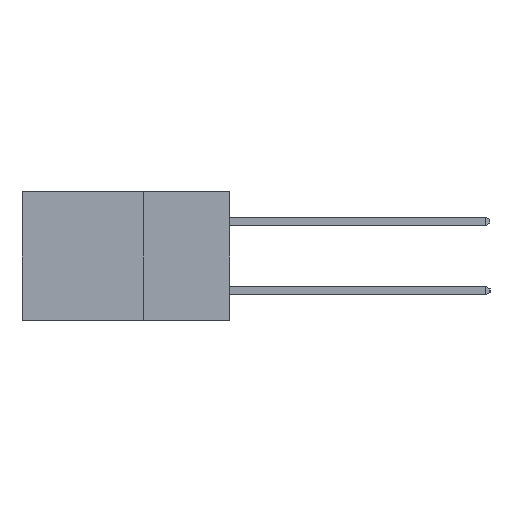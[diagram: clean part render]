
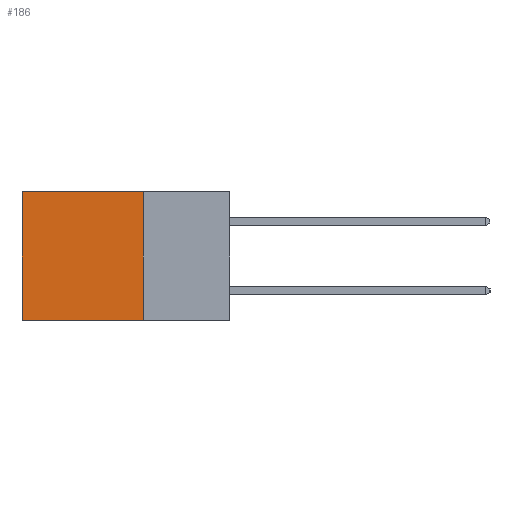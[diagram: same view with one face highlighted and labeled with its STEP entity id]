
A CAD part, left-side view. The second image highlights one B-rep face of the part: STEP entity #186.
In plain terms, the highlighted planar face has unit normal (-1, 0, 0).
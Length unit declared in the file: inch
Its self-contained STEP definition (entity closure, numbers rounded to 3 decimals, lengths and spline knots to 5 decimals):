
#186 = ADVANCED_FACE ( 'NONE', ( #10603 ), #6259, .F. ) ;
#323 = DIRECTION ( 'NONE',  ( 1., 0., 0. ) ) ;
#599 = ORIENTED_EDGE ( 'NONE', *, *, #1498, .F. ) ;
#698 = CARTESIAN_POINT ( 'NONE',  ( 0.2615, 0.6, -0.37 ) ) ;
#820 = EDGE_CURVE ( 'NONE', #10385, #2219, #7479, .T. ) ;
#920 = ORIENTED_EDGE ( 'NONE', *, *, #12035, .F. ) ;
#1498 = EDGE_CURVE ( 'NONE', #5445, #3786, #5618, .T. ) ;
#1871 = VECTOR ( 'NONE', #5657, 39.37008 ) ;
#2219 = VERTEX_POINT ( 'NONE', #8267 ) ;
#2277 = DIRECTION ( 'NONE',  ( 0., 1., 0. ) ) ;
#2538 = EDGE_CURVE ( 'NONE', #2219, #3786, #9762, .T. ) ;
#2565 = VECTOR ( 'NONE', #3192, 39.37008 ) ;
#3192 = DIRECTION ( 'NONE',  ( 0., 0., -1. ) ) ;
#3281 = CARTESIAN_POINT ( 'NONE',  ( 0.2615, 0.25, -0.37 ) ) ;
#3577 = EDGE_LOOP ( 'NONE', ( #4895, #599, #920, #8936 ) ) ;
#3672 = CARTESIAN_POINT ( 'NONE',  ( 0.2615, 0.25, -0.37 ) ) ;
#3786 = VERTEX_POINT ( 'NONE', #4254 ) ;
#4254 = CARTESIAN_POINT ( 'NONE',  ( 0.2615, 0.6, -0.37 ) ) ;
#4895 = ORIENTED_EDGE ( 'NONE', *, *, #2538, .T. ) ;
#5445 = VERTEX_POINT ( 'NONE', #3672 ) ;
#5578 = CARTESIAN_POINT ( 'NONE',  ( 0.2615, 0.25, 0. ) ) ;
#5618 = LINE ( 'NONE', #3281, #10561 ) ;
#5657 = DIRECTION ( 'NONE',  ( 0., 0., -1. ) ) ;
#6259 = PLANE ( 'NONE',  #7540 ) ;
#7237 = DIRECTION ( 'NONE',  ( 0., 0., -1. ) ) ;
#7479 = LINE ( 'NONE', #10162, #12457 ) ;
#7540 = AXIS2_PLACEMENT_3D ( 'NONE', #11194, #323, #7237 ) ;
#8267 = CARTESIAN_POINT ( 'NONE',  ( 0.2615, 0.6, 0. ) ) ;
#8936 = ORIENTED_EDGE ( 'NONE', *, *, #820, .T. ) ;
#9762 = LINE ( 'NONE', #698, #1871 ) ;
#10111 = CARTESIAN_POINT ( 'NONE',  ( 0.2615, 0.25, -0.37 ) ) ;
#10136 = LINE ( 'NONE', #10111, #2565 ) ;
#10162 = CARTESIAN_POINT ( 'NONE',  ( 0.2615, 0.25, 0. ) ) ;
#10385 = VERTEX_POINT ( 'NONE', #5578 ) ;
#10561 = VECTOR ( 'NONE', #2277, 39.37008 ) ;
#10603 = FACE_OUTER_BOUND ( 'NONE', #3577, .T. ) ;
#11168 = DIRECTION ( 'NONE',  ( 0., 1., 0. ) ) ;
#11194 = CARTESIAN_POINT ( 'NONE',  ( 0.2615, 0.25, -0.37 ) ) ;
#12035 = EDGE_CURVE ( 'NONE', #10385, #5445, #10136, .T. ) ;
#12457 = VECTOR ( 'NONE', #11168, 39.37008 ) ;
